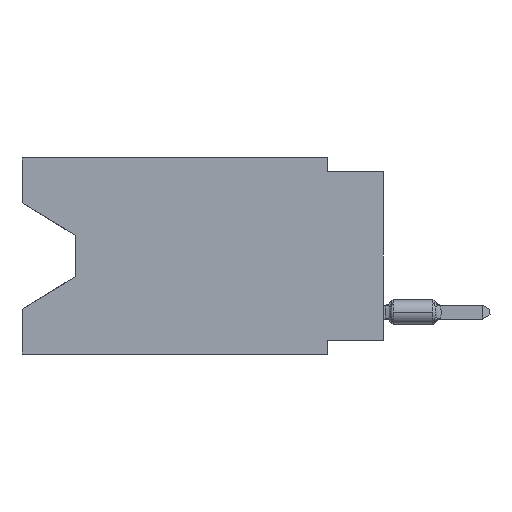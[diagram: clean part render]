
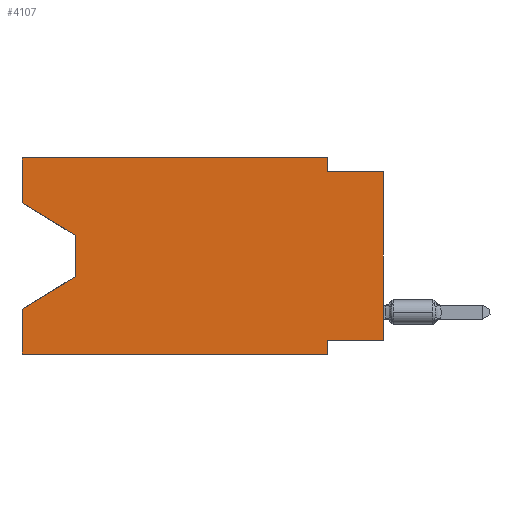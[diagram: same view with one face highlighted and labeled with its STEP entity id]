
A CAD part, left-side view. The second image highlights one B-rep face of the part: STEP entity #4107.
In plain terms, the highlighted planar face has unit normal (-1, 0, 0).
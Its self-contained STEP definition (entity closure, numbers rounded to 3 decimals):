
#85 = ORIENTED_EDGE ( 'NONE', *, *, #12960, .T. ) ;
#132 = VECTOR ( 'NONE', #4934, 1000. ) ;
#190 = ORIENTED_EDGE ( 'NONE', *, *, #10656, .F. ) ;
#214 = EDGE_CURVE ( 'NONE', #10856, #8486, #1797, .T. ) ;
#220 = VECTOR ( 'NONE', #4505, 1000. ) ;
#367 = VECTOR ( 'NONE', #6029, 1000. ) ;
#490 = DIRECTION ( 'NONE',  ( 0., 0., 1. ) ) ;
#533 = LINE ( 'NONE', #6819, #3691 ) ;
#833 = CARTESIAN_POINT ( 'NONE',  ( 0., 16.383, 0. ) ) ;
#930 = CARTESIAN_POINT ( 'NONE',  ( 0., 2.54, -8.255 ) ) ;
#1013 = VECTOR ( 'NONE', #9763, 1000. ) ;
#1271 = ORIENTED_EDGE ( 'NONE', *, *, #4028, .T. ) ;
#1310 = VECTOR ( 'NONE', #6692, 1000. ) ;
#1504 = LINE ( 'NONE', #5818, #3442 ) ;
#1568 = CARTESIAN_POINT ( 'NONE',  ( 0., 13.97, -3.505 ) ) ;
#1584 = CARTESIAN_POINT ( 'NONE',  ( 0., 2.54, -8.89 ) ) ;
#1797 = LINE ( 'NONE', #1933, #8783 ) ;
#1933 = CARTESIAN_POINT ( 'NONE',  ( 0., 0., -0.635 ) ) ;
#2025 = CARTESIAN_POINT ( 'NONE',  ( 0., 2.54, 0. ) ) ;
#2244 = VERTEX_POINT ( 'NONE', #1584 ) ;
#2301 = DIRECTION ( 'NONE',  ( 0., 0., -1. ) ) ;
#2343 = EDGE_CURVE ( 'NONE', #10966, #4919, #7186, .T. ) ;
#2420 = VECTOR ( 'NONE', #5331, 1000. ) ;
#2586 = EDGE_CURVE ( 'NONE', #13150, #11728, #1504, .T. ) ;
#2655 = ORIENTED_EDGE ( 'NONE', *, *, #4723, .T. ) ;
#2837 = CARTESIAN_POINT ( 'NONE',  ( 0., 16.383, -8.89 ) ) ;
#2954 = CARTESIAN_POINT ( 'NONE',  ( 0., 0., -8.255 ) ) ;
#3070 = VECTOR ( 'NONE', #7782, 1000. ) ;
#3107 = VERTEX_POINT ( 'NONE', #12213 ) ;
#3442 = VECTOR ( 'NONE', #490, 1000. ) ;
#3620 = CARTESIAN_POINT ( 'NONE',  ( 0., 13.97, -3.505 ) ) ;
#3671 = ORIENTED_EDGE ( 'NONE', *, *, #7704, .F. ) ;
#3691 = VECTOR ( 'NONE', #9581, 1000. ) ;
#3822 = EDGE_CURVE ( 'NONE', #13150, #2244, #3910, .T. ) ;
#3839 = FACE_OUTER_BOUND ( 'NONE', #6996, .T. ) ;
#3854 = CARTESIAN_POINT ( 'NONE',  ( 0., 16.383, 0. ) ) ;
#3910 = LINE ( 'NONE', #2837, #12307 ) ;
#4028 = EDGE_CURVE ( 'NONE', #11164, #11728, #533, .T. ) ;
#4086 = VERTEX_POINT ( 'NONE', #930 ) ;
#4107 = ADVANCED_FACE ( 'NONE', ( #3839 ), #11051, .F. ) ;
#4505 = DIRECTION ( 'NONE',  ( 0., -0.855, -0.519 ) ) ;
#4723 = EDGE_CURVE ( 'NONE', #9561, #11164, #4811, .T. ) ;
#4811 = LINE ( 'NONE', #1568, #3070 ) ;
#4879 = CARTESIAN_POINT ( 'NONE',  ( 0., 13.97, -5.385 ) ) ;
#4919 = VERTEX_POINT ( 'NONE', #3854 ) ;
#4934 = DIRECTION ( 'NONE',  ( 0., 1., 0. ) ) ;
#5057 = DIRECTION ( 'NONE',  ( 1., 0., 0. ) ) ;
#5331 = DIRECTION ( 'NONE',  ( 0., 0., -1. ) ) ;
#5470 = LINE ( 'NONE', #11536, #6656 ) ;
#5739 = CARTESIAN_POINT ( 'NONE',  ( 0., 16.383, 0. ) ) ;
#5798 = DIRECTION ( 'NONE',  ( 0., -1., 0. ) ) ;
#5818 = CARTESIAN_POINT ( 'NONE',  ( 0., 16.383, 0. ) ) ;
#6029 = DIRECTION ( 'NONE',  ( 0., 0., 1. ) ) ;
#6037 = EDGE_CURVE ( 'NONE', #10966, #9561, #6588, .T. ) ;
#6257 = EDGE_CURVE ( 'NONE', #4919, #3107, #12767, .T. ) ;
#6505 = ORIENTED_EDGE ( 'NONE', *, *, #2343, .F. ) ;
#6588 = LINE ( 'NONE', #7609, #220 ) ;
#6656 = VECTOR ( 'NONE', #2301, 1000. ) ;
#6692 = DIRECTION ( 'NONE',  ( 0., -1., 0. ) ) ;
#6819 = CARTESIAN_POINT ( 'NONE',  ( 0., 13.97, -5.385 ) ) ;
#6996 = EDGE_LOOP ( 'NONE', ( #8019, #2655, #1271, #12661, #13349, #190, #7420, #85, #7521, #3671, #10854, #6505 ) ) ;
#7093 = CARTESIAN_POINT ( 'NONE',  ( 0., 0., -8.255 ) ) ;
#7186 = LINE ( 'NONE', #833, #367 ) ;
#7420 = ORIENTED_EDGE ( 'NONE', *, *, #12159, .F. ) ;
#7521 = ORIENTED_EDGE ( 'NONE', *, *, #214, .F. ) ;
#7609 = CARTESIAN_POINT ( 'NONE',  ( 0., 16.383, -2.038 ) ) ;
#7704 = EDGE_CURVE ( 'NONE', #3107, #10856, #12346, .T. ) ;
#7738 = CARTESIAN_POINT ( 'NONE',  ( 0., 0., -0.635 ) ) ;
#7782 = DIRECTION ( 'NONE',  ( 0., 0., -1. ) ) ;
#8019 = ORIENTED_EDGE ( 'NONE', *, *, #6037, .T. ) ;
#8142 = CARTESIAN_POINT ( 'NONE',  ( 0., 16.383, -8.89 ) ) ;
#8486 = VERTEX_POINT ( 'NONE', #7738 ) ;
#8783 = VECTOR ( 'NONE', #10909, 1000. ) ;
#9561 = VERTEX_POINT ( 'NONE', #3620 ) ;
#9581 = DIRECTION ( 'NONE',  ( 0., 0.855, -0.519 ) ) ;
#9730 = AXIS2_PLACEMENT_3D ( 'NONE', #11115, #5057, #12074 ) ;
#9763 = DIRECTION ( 'NONE',  ( 0., 0., 1. ) ) ;
#10201 = CARTESIAN_POINT ( 'NONE',  ( 0., 16.383, -6.852 ) ) ;
#10656 = EDGE_CURVE ( 'NONE', #4086, #2244, #5470, .T. ) ;
#10854 = ORIENTED_EDGE ( 'NONE', *, *, #6257, .F. ) ;
#10856 = VERTEX_POINT ( 'NONE', #11045 ) ;
#10909 = DIRECTION ( 'NONE',  ( 0., -1., 0. ) ) ;
#10966 = VERTEX_POINT ( 'NONE', #11704 ) ;
#11045 = CARTESIAN_POINT ( 'NONE',  ( 0., 2.54, -0.635 ) ) ;
#11051 = PLANE ( 'NONE',  #9730 ) ;
#11115 = CARTESIAN_POINT ( 'NONE',  ( 0., 16.383, 0. ) ) ;
#11164 = VERTEX_POINT ( 'NONE', #4879 ) ;
#11536 = CARTESIAN_POINT ( 'NONE',  ( 0., 2.54, -8.89 ) ) ;
#11704 = CARTESIAN_POINT ( 'NONE',  ( 0., 16.383, -2.038 ) ) ;
#11728 = VERTEX_POINT ( 'NONE', #10201 ) ;
#12074 = DIRECTION ( 'NONE',  ( 0., 0., -1. ) ) ;
#12159 = EDGE_CURVE ( 'NONE', #12792, #4086, #12769, .T. ) ;
#12213 = CARTESIAN_POINT ( 'NONE',  ( 0., 2.54, 0. ) ) ;
#12307 = VECTOR ( 'NONE', #5798, 1000. ) ;
#12346 = LINE ( 'NONE', #2025, #2420 ) ;
#12661 = ORIENTED_EDGE ( 'NONE', *, *, #2586, .F. ) ;
#12671 = LINE ( 'NONE', #12800, #1013 ) ;
#12767 = LINE ( 'NONE', #5739, #1310 ) ;
#12769 = LINE ( 'NONE', #7093, #132 ) ;
#12792 = VERTEX_POINT ( 'NONE', #2954 ) ;
#12800 = CARTESIAN_POINT ( 'NONE',  ( 0., 0., 0. ) ) ;
#12960 = EDGE_CURVE ( 'NONE', #12792, #8486, #12671, .T. ) ;
#13150 = VERTEX_POINT ( 'NONE', #8142 ) ;
#13349 = ORIENTED_EDGE ( 'NONE', *, *, #3822, .T. ) ;
